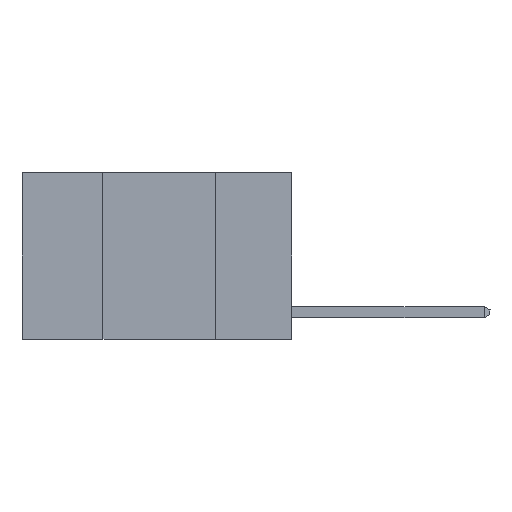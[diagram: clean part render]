
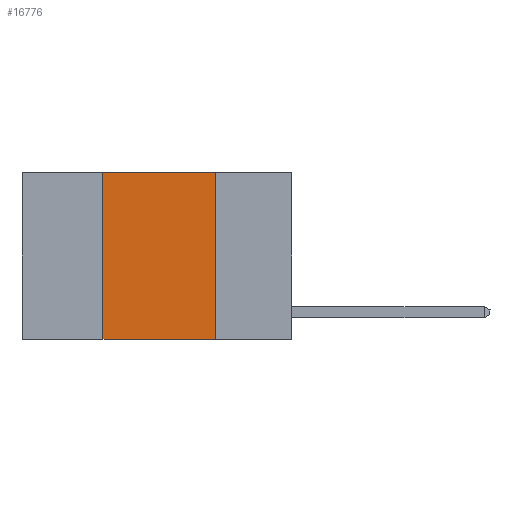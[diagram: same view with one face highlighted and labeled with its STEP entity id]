
A CAD part, left-side view. The second image highlights one B-rep face of the part: STEP entity #16776.
In plain terms, the highlighted planar face has unit normal (-1, 0, 0).
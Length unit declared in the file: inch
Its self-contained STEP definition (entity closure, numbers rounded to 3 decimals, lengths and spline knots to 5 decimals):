
#36 = DIRECTION ( 'NONE',  ( 1., 0., 0. ) ) ;
#208 = AXIS2_PLACEMENT_3D ( 'NONE', #22049, #36, #13006 ) ;
#1528 = EDGE_CURVE ( 'NONE', #10958, #5506, #19986, .T. ) ;
#2560 = VERTEX_POINT ( 'NONE', #14645 ) ;
#2775 = EDGE_CURVE ( 'NONE', #10958, #7666, #11987, .T. ) ;
#3500 = DIRECTION ( 'NONE',  ( 0., -1., 0. ) ) ;
#3790 = EDGE_CURVE ( 'NONE', #5506, #2560, #13688, .T. ) ;
#3938 = EDGE_CURVE ( 'NONE', #2560, #7666, #19297, .T. ) ;
#4594 = DIRECTION ( 'NONE',  ( 0., 0., 1. ) ) ;
#5506 = VERTEX_POINT ( 'NONE', #7974 ) ;
#5529 = ORIENTED_EDGE ( 'NONE', *, *, #3938, .F. ) ;
#5758 = DIRECTION ( 'NONE',  ( 0., 0., -1. ) ) ;
#6131 = CARTESIAN_POINT ( 'NONE',  ( 0., 0.6, -0.37 ) ) ;
#7037 = VECTOR ( 'NONE', #20817, 39.37008 ) ;
#7666 = VERTEX_POINT ( 'NONE', #23539 ) ;
#7974 = CARTESIAN_POINT ( 'NONE',  ( 0., 0.42, 0. ) ) ;
#8182 = VECTOR ( 'NONE', #3500, 39.37008 ) ;
#8211 = EDGE_LOOP ( 'NONE', ( #5529, #10500, #11087, #20751 ) ) ;
#10500 = ORIENTED_EDGE ( 'NONE', *, *, #3790, .F. ) ;
#10918 = VECTOR ( 'NONE', #4594, 39.37008 ) ;
#10958 = VERTEX_POINT ( 'NONE', #21604 ) ;
#11087 = ORIENTED_EDGE ( 'NONE', *, *, #1528, .F. ) ;
#11987 = LINE ( 'NONE', #6131, #7037 ) ;
#12740 = FACE_OUTER_BOUND ( 'NONE', #8211, .T. ) ;
#13006 = DIRECTION ( 'NONE',  ( 0., 0., -1. ) ) ;
#13151 = CARTESIAN_POINT ( 'NONE',  ( 0., 0.17, 0. ) ) ;
#13688 = LINE ( 'NONE', #23634, #8182 ) ;
#14645 = CARTESIAN_POINT ( 'NONE',  ( 0., 0.17, 0. ) ) ;
#16776 = ADVANCED_FACE ( 'NONE', ( #12740 ), #20218, .F. ) ;
#17408 = CARTESIAN_POINT ( 'NONE',  ( 0., 0.42, 0. ) ) ;
#19297 = LINE ( 'NONE', #13151, #23615 ) ;
#19986 = LINE ( 'NONE', #17408, #10918 ) ;
#20218 = PLANE ( 'NONE',  #208 ) ;
#20751 = ORIENTED_EDGE ( 'NONE', *, *, #2775, .T. ) ;
#20817 = DIRECTION ( 'NONE',  ( 0., -1., 0. ) ) ;
#21604 = CARTESIAN_POINT ( 'NONE',  ( 0., 0.42, -0.37 ) ) ;
#22049 = CARTESIAN_POINT ( 'NONE',  ( 0., 0.6, 0. ) ) ;
#23539 = CARTESIAN_POINT ( 'NONE',  ( 0., 0.17, -0.37 ) ) ;
#23615 = VECTOR ( 'NONE', #5758, 39.37008 ) ;
#23634 = CARTESIAN_POINT ( 'NONE',  ( 0., 0.6, 0. ) ) ;
